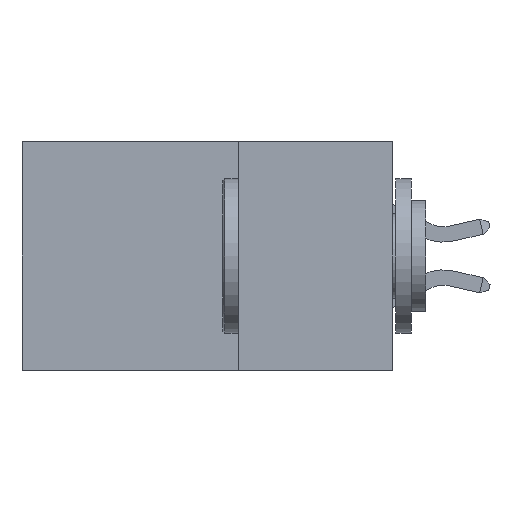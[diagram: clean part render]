
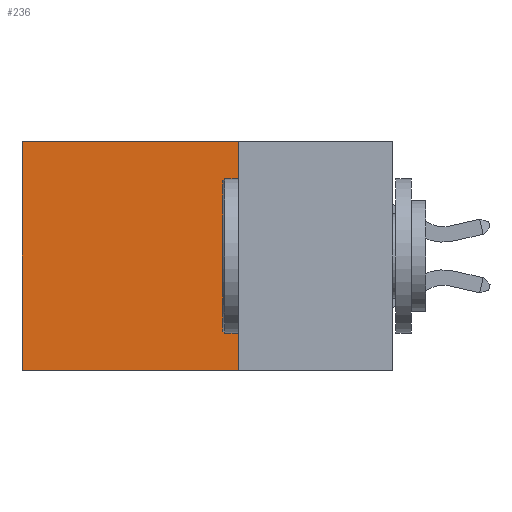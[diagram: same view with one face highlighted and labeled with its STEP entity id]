
A CAD part, left-side view. The second image highlights one B-rep face of the part: STEP entity #236.
In plain terms, the highlighted planar face has unit normal (-1, 0, 0).
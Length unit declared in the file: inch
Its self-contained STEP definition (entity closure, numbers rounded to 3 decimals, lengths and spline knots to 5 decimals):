
#236 = ADVANCED_FACE ( 'NONE', ( #13235 ), #15906, .F. ) ;
#1255 = VECTOR ( 'NONE', #13063, 39.37008 ) ;
#3561 = VECTOR ( 'NONE', #13005, 39.37008 ) ;
#4036 = VECTOR ( 'NONE', #6085, 39.37008 ) ;
#5466 = DIRECTION ( 'NONE',  ( 0., 1., 0. ) ) ;
#6085 = DIRECTION ( 'NONE',  ( 0., 1., 0. ) ) ;
#7479 = EDGE_CURVE ( 'NONE', #13076, #11625, #15123, .T. ) ;
#7910 = EDGE_CURVE ( 'NONE', #14155, #13076, #11936, .T. ) ;
#8094 = VERTEX_POINT ( 'NONE', #15878 ) ;
#8191 = CARTESIAN_POINT ( 'NONE',  ( 0.2875, 0.6, -0.37 ) ) ;
#8323 = ORIENTED_EDGE ( 'NONE', *, *, #12354, .F. ) ;
#9884 = CARTESIAN_POINT ( 'NONE',  ( 0.2875, 0.25, 0. ) ) ;
#11416 = CARTESIAN_POINT ( 'NONE',  ( 0.2875, 0.6, 0. ) ) ;
#11468 = CARTESIAN_POINT ( 'NONE',  ( 0.2875, 0.25, 0. ) ) ;
#11625 = VERTEX_POINT ( 'NONE', #8191 ) ;
#11753 = CARTESIAN_POINT ( 'NONE',  ( 0.2875, 0.25, -0.37 ) ) ;
#11936 = LINE ( 'NONE', #13941, #4036 ) ;
#12354 = EDGE_CURVE ( 'NONE', #14155, #8094, #18399, .T. ) ;
#12440 = AXIS2_PLACEMENT_3D ( 'NONE', #15579, #15454, #15430 ) ;
#13005 = DIRECTION ( 'NONE',  ( 0., 0., -1. ) ) ;
#13063 = DIRECTION ( 'NONE',  ( 0., 0., -1. ) ) ;
#13076 = VERTEX_POINT ( 'NONE', #19531 ) ;
#13235 = FACE_OUTER_BOUND ( 'NONE', #18713, .T. ) ;
#13941 = CARTESIAN_POINT ( 'NONE',  ( 0.2875, 0.25, 0. ) ) ;
#14155 = VERTEX_POINT ( 'NONE', #9884 ) ;
#14984 = LINE ( 'NONE', #11753, #18557 ) ;
#15123 = LINE ( 'NONE', #11416, #3561 ) ;
#15185 = ORIENTED_EDGE ( 'NONE', *, *, #17507, .F. ) ;
#15430 = DIRECTION ( 'NONE',  ( 0., 0., -1. ) ) ;
#15454 = DIRECTION ( 'NONE',  ( 1., 0., 0. ) ) ;
#15579 = CARTESIAN_POINT ( 'NONE',  ( 0.2875, 0.25, 0. ) ) ;
#15878 = CARTESIAN_POINT ( 'NONE',  ( 0.2875, 0.25, -0.37 ) ) ;
#15906 = PLANE ( 'NONE',  #12440 ) ;
#17507 = EDGE_CURVE ( 'NONE', #8094, #11625, #14984, .T. ) ;
#17584 = ORIENTED_EDGE ( 'NONE', *, *, #7910, .T. ) ;
#18399 = LINE ( 'NONE', #11468, #1255 ) ;
#18557 = VECTOR ( 'NONE', #5466, 39.37008 ) ;
#18713 = EDGE_LOOP ( 'NONE', ( #19638, #15185, #8323, #17584 ) ) ;
#19531 = CARTESIAN_POINT ( 'NONE',  ( 0.2875, 0.6, 0. ) ) ;
#19638 = ORIENTED_EDGE ( 'NONE', *, *, #7479, .T. ) ;
